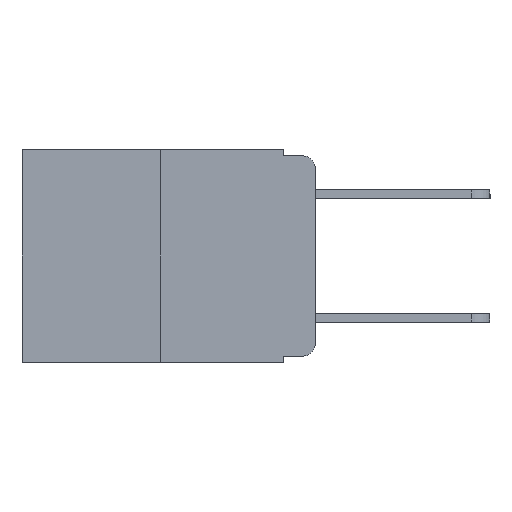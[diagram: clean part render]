
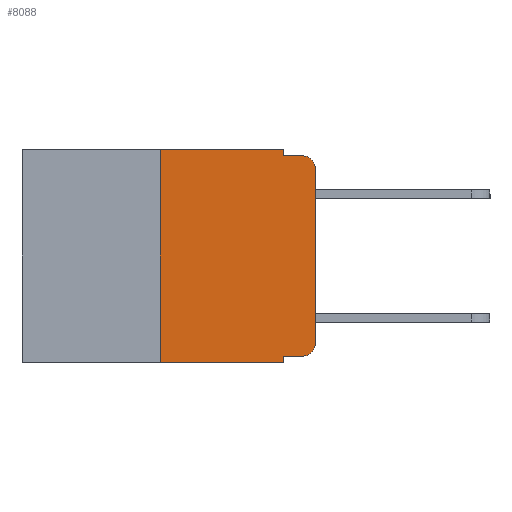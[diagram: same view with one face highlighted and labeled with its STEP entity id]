
A CAD part, left-side view. The second image highlights one B-rep face of the part: STEP entity #8088.
In plain terms, the highlighted planar face has unit normal (-1, 0, 0).
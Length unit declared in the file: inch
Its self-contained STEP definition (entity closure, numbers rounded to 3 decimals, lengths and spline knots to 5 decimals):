
#34 = VERTEX_POINT ( 'NONE', #4577 ) ;
#96 = DIRECTION ( 'NONE',  ( 0., 0., 1. ) ) ;
#216 = EDGE_CURVE ( 'NONE', #2423, #4139, #10900, .T. ) ;
#369 = PLANE ( 'NONE',  #9684 ) ;
#374 = CIRCLE ( 'NONE', #9444, 0.02 ) ;
#717 = VERTEX_POINT ( 'NONE', #3853 ) ;
#744 = DIRECTION ( 'NONE',  ( 0., -1., 0. ) ) ;
#809 = CARTESIAN_POINT ( 'NONE',  ( 0., 0., -0.03 ) ) ;
#1021 = LINE ( 'NONE', #7540, #10114 ) ;
#1784 = VERTEX_POINT ( 'NONE', #6107 ) ;
#2035 = EDGE_CURVE ( 'NONE', #4139, #8101, #374, .T. ) ;
#2041 = VECTOR ( 'NONE', #8318, 39.37008 ) ;
#2081 = EDGE_CURVE ( 'NONE', #4807, #34, #2386, .T. ) ;
#2112 = CARTESIAN_POINT ( 'NONE',  ( 0., 0.051, -0.333 ) ) ;
#2264 = DIRECTION ( 'NONE',  ( 0., 0., -1. ) ) ;
#2386 = LINE ( 'NONE', #10233, #5143 ) ;
#2423 = VERTEX_POINT ( 'NONE', #2849 ) ;
#2490 = VERTEX_POINT ( 'NONE', #11264 ) ;
#2699 = DIRECTION ( 'NONE',  ( 0., 0., -1. ) ) ;
#2805 = VERTEX_POINT ( 'NONE', #809 ) ;
#2849 = CARTESIAN_POINT ( 'NONE',  ( 0., 0.051, -0.333 ) ) ;
#3367 = CARTESIAN_POINT ( 'NONE',  ( 0., 0.051, 0. ) ) ;
#3441 = LINE ( 'NONE', #3782, #7613 ) ;
#3782 = CARTESIAN_POINT ( 'NONE',  ( 0., 0.25, 0. ) ) ;
#3853 = CARTESIAN_POINT ( 'NONE',  ( 0., 0.02, -0.01 ) ) ;
#4051 = EDGE_LOOP ( 'NONE', ( #5358, #5280, #5265, #5195, #5203, #5002, #4847, #4793, #4744, #10356 ) ) ;
#4139 = VERTEX_POINT ( 'NONE', #8801 ) ;
#4325 = CARTESIAN_POINT ( 'NONE',  ( 0., 0.02, -0.03 ) ) ;
#4433 = CARTESIAN_POINT ( 'NONE',  ( 0., 0.473, -0.343 ) ) ;
#4577 = CARTESIAN_POINT ( 'NONE',  ( 0., 0.051, 0. ) ) ;
#4742 = FACE_OUTER_BOUND ( 'NONE', #4051, .T. ) ;
#4744 = ORIENTED_EDGE ( 'NONE', *, *, #216, .T. ) ;
#4793 = ORIENTED_EDGE ( 'NONE', *, *, #9145, .F. ) ;
#4807 = VERTEX_POINT ( 'NONE', #9431 ) ;
#4847 = ORIENTED_EDGE ( 'NONE', *, *, #6198, .T. ) ;
#5002 = ORIENTED_EDGE ( 'NONE', *, *, #10013, .F. ) ;
#5143 = VECTOR ( 'NONE', #8753, 39.37008 ) ;
#5151 = DIRECTION ( 'NONE',  ( 0., 0., -1. ) ) ;
#5195 = ORIENTED_EDGE ( 'NONE', *, *, #11124, .F. ) ;
#5203 = ORIENTED_EDGE ( 'NONE', *, *, #2081, .F. ) ;
#5265 = ORIENTED_EDGE ( 'NONE', *, *, #6249, .F. ) ;
#5280 = ORIENTED_EDGE ( 'NONE', *, *, #6123, .T. ) ;
#5358 = ORIENTED_EDGE ( 'NONE', *, *, #6155, .T. ) ;
#5539 = VECTOR ( 'NONE', #96, 39.37008 ) ;
#5802 = LINE ( 'NONE', #10754, #5539 ) ;
#6107 = CARTESIAN_POINT ( 'NONE',  ( 0., 0.051, -0.01 ) ) ;
#6123 = EDGE_CURVE ( 'NONE', #2805, #717, #6561, .T. ) ;
#6155 = EDGE_CURVE ( 'NONE', #8101, #2805, #5802, .T. ) ;
#6198 = EDGE_CURVE ( 'NONE', #2490, #10707, #7202, .T. ) ;
#6234 = CARTESIAN_POINT ( 'NONE',  ( 0., 0.473, 0. ) ) ;
#6249 = EDGE_CURVE ( 'NONE', #1784, #717, #8519, .T. ) ;
#6422 = VECTOR ( 'NONE', #7738, 39.37008 ) ;
#6523 = DIRECTION ( 'NONE',  ( 0., 0., -1. ) ) ;
#6561 = CIRCLE ( 'NONE', #8854, 0.02 ) ;
#6564 = DIRECTION ( 'NONE',  ( -1., 0., 0. ) ) ;
#6619 = CARTESIAN_POINT ( 'NONE',  ( 0., 0.02, -0.313 ) ) ;
#6857 = LINE ( 'NONE', #3367, #2041 ) ;
#6960 = CARTESIAN_POINT ( 'NONE',  ( 0., 0.051, -0.01 ) ) ;
#7202 = LINE ( 'NONE', #4433, #11072 ) ;
#7540 = CARTESIAN_POINT ( 'NONE',  ( 0., 0.051, 0. ) ) ;
#7613 = VECTOR ( 'NONE', #11005, 39.37008 ) ;
#7738 = DIRECTION ( 'NONE',  ( 0., -1., 0. ) ) ;
#7821 = DIRECTION ( 'NONE',  ( 1., 0., 0. ) ) ;
#8088 = ADVANCED_FACE ( 'NONE', ( #4742 ), #369, .F. ) ;
#8101 = VERTEX_POINT ( 'NONE', #10949 ) ;
#8318 = DIRECTION ( 'NONE',  ( 0., 0., -1. ) ) ;
#8458 = DIRECTION ( 'NONE',  ( 0., -1., 0. ) ) ;
#8519 = LINE ( 'NONE', #6960, #6422 ) ;
#8753 = DIRECTION ( 'NONE',  ( 0., -1., 0. ) ) ;
#8801 = CARTESIAN_POINT ( 'NONE',  ( 0., 0.02, -0.333 ) ) ;
#8854 = AXIS2_PLACEMENT_3D ( 'NONE', #4325, #9983, #5151 ) ;
#9145 = EDGE_CURVE ( 'NONE', #2423, #10707, #1021, .T. ) ;
#9431 = CARTESIAN_POINT ( 'NONE',  ( 0., 0.25, 0. ) ) ;
#9444 = AXIS2_PLACEMENT_3D ( 'NONE', #6619, #6564, #6523 ) ;
#9684 = AXIS2_PLACEMENT_3D ( 'NONE', #6234, #7821, #2699 ) ;
#9983 = DIRECTION ( 'NONE',  ( -1., 0., 0. ) ) ;
#10013 = EDGE_CURVE ( 'NONE', #2490, #4807, #3441, .T. ) ;
#10114 = VECTOR ( 'NONE', #2264, 39.37008 ) ;
#10233 = CARTESIAN_POINT ( 'NONE',  ( 0., 0.473, 0. ) ) ;
#10356 = ORIENTED_EDGE ( 'NONE', *, *, #2035, .T. ) ;
#10681 = VECTOR ( 'NONE', #744, 39.37008 ) ;
#10707 = VERTEX_POINT ( 'NONE', #11001 ) ;
#10754 = CARTESIAN_POINT ( 'NONE',  ( 0., 0., 0. ) ) ;
#10900 = LINE ( 'NONE', #2112, #10681 ) ;
#10949 = CARTESIAN_POINT ( 'NONE',  ( 0., 0., -0.313 ) ) ;
#11001 = CARTESIAN_POINT ( 'NONE',  ( 0., 0.051, -0.343 ) ) ;
#11005 = DIRECTION ( 'NONE',  ( 0., 0., 1. ) ) ;
#11072 = VECTOR ( 'NONE', #8458, 39.37008 ) ;
#11124 = EDGE_CURVE ( 'NONE', #34, #1784, #6857, .T. ) ;
#11264 = CARTESIAN_POINT ( 'NONE',  ( 0., 0.25, -0.343 ) ) ;
